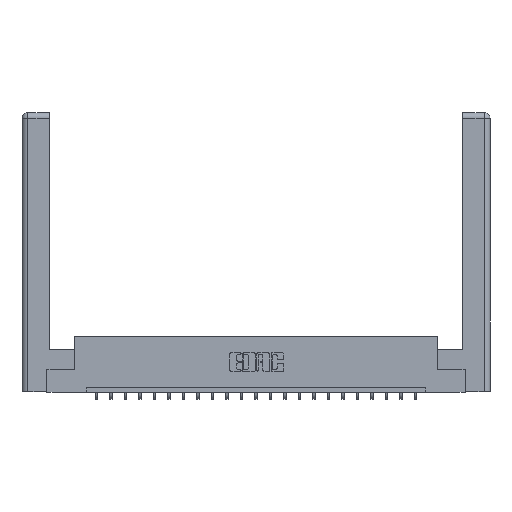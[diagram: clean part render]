
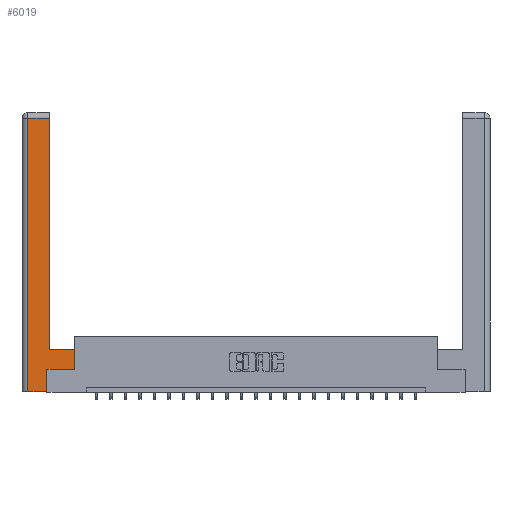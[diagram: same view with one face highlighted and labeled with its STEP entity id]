
A CAD part, top view. The second image highlights one B-rep face of the part: STEP entity #6019.
In plain terms, the highlighted planar face has unit normal (0, 0, 1).
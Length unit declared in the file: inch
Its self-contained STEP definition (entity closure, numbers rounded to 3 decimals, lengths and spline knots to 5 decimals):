
#925 = CARTESIAN_POINT ( 'NONE',  ( 0., 0., 0. ) ) ;
#1582 = EDGE_CURVE ( 'NONE', #2678, #2414, #10447, .T. ) ;
#1807 = ORIENTED_EDGE ( 'NONE', *, *, #10558, .T. ) ;
#2045 = CARTESIAN_POINT ( 'NONE',  ( 0.295, 0.45, 0. ) ) ;
#2333 = VECTOR ( 'NONE', #15554, 39.37008 ) ;
#2414 = VERTEX_POINT ( 'NONE', #6333 ) ;
#2653 = EDGE_CURVE ( 'NONE', #2414, #18316, #16568, .T. ) ;
#2678 = VERTEX_POINT ( 'NONE', #7148 ) ;
#3424 = DIRECTION ( 'NONE',  ( 0., 1., 0. ) ) ;
#3542 = CARTESIAN_POINT ( 'NONE',  ( 0.295, 0.45, 0. ) ) ;
#3583 = DIRECTION ( 'NONE',  ( -1., 0., 0. ) ) ;
#4177 = LINE ( 'NONE', #17579, #14940 ) ;
#4612 = LINE ( 'NONE', #7043, #17806 ) ;
#5294 = EDGE_CURVE ( 'NONE', #15236, #6490, #16550, .T. ) ;
#5371 = EDGE_CURVE ( 'NONE', #18316, #11272, #4177, .T. ) ;
#6019 = ADVANCED_FACE ( 'NONE', ( #17327 ), #9470, .F. ) ;
#6333 = CARTESIAN_POINT ( 'NONE',  ( 0.565, 0.45, 0. ) ) ;
#6456 = ORIENTED_EDGE ( 'NONE', *, *, #5294, .T. ) ;
#6490 = VERTEX_POINT ( 'NONE', #19082 ) ;
#7034 = ORIENTED_EDGE ( 'NONE', *, *, #5371, .T. ) ;
#7043 = CARTESIAN_POINT ( 'NONE',  ( 0.565, 0.245, 0. ) ) ;
#7148 = CARTESIAN_POINT ( 'NONE',  ( 0.565, 0.245, 0. ) ) ;
#7557 = EDGE_CURVE ( 'NONE', #6490, #10489, #11577, .T. ) ;
#7897 = DIRECTION ( 'NONE',  ( -1., 0., 0. ) ) ;
#8452 = CARTESIAN_POINT ( 'NONE',  ( 0.0615, 2.94, 0. ) ) ;
#8713 = DIRECTION ( 'NONE',  ( 1., 0., 0. ) ) ;
#8998 = LINE ( 'NONE', #10266, #11144 ) ;
#9437 = VECTOR ( 'NONE', #15833, 39.37008 ) ;
#9470 = PLANE ( 'NONE',  #16170 ) ;
#10266 = CARTESIAN_POINT ( 'NONE',  ( 0.0615, 2.94, 0. ) ) ;
#10368 = VECTOR ( 'NONE', #16097, 39.37008 ) ;
#10447 = LINE ( 'NONE', #20056, #20625 ) ;
#10489 = VERTEX_POINT ( 'NONE', #15449 ) ;
#10558 = EDGE_CURVE ( 'NONE', #11272, #13609, #8998, .T. ) ;
#11144 = VECTOR ( 'NONE', #3583, 39.37008 ) ;
#11272 = VERTEX_POINT ( 'NONE', #19747 ) ;
#11407 = ORIENTED_EDGE ( 'NONE', *, *, #16576, .T. ) ;
#11577 = LINE ( 'NONE', #21186, #9437 ) ;
#13609 = VERTEX_POINT ( 'NONE', #8452 ) ;
#14940 = VECTOR ( 'NONE', #21042, 39.37008 ) ;
#15011 = DIRECTION ( 'NONE',  ( 0., -1., 0. ) ) ;
#15236 = VERTEX_POINT ( 'NONE', #18381 ) ;
#15449 = CARTESIAN_POINT ( 'NONE',  ( 0.265, 0.245, 0. ) ) ;
#15554 = DIRECTION ( 'NONE',  ( -1., 0., 0. ) ) ;
#15833 = DIRECTION ( 'NONE',  ( 0., 1., 0. ) ) ;
#15844 = EDGE_CURVE ( 'NONE', #10489, #2678, #4612, .T. ) ;
#16097 = DIRECTION ( 'NONE',  ( 1., 0., 0. ) ) ;
#16170 = AXIS2_PLACEMENT_3D ( 'NONE', #925, #21529, #7897 ) ;
#16186 = ORIENTED_EDGE ( 'NONE', *, *, #2653, .T. ) ;
#16550 = LINE ( 'NONE', #18359, #10368 ) ;
#16568 = LINE ( 'NONE', #3542, #2333 ) ;
#16576 = EDGE_CURVE ( 'NONE', #13609, #15236, #21809, .T. ) ;
#17061 = ORIENTED_EDGE ( 'NONE', *, *, #1582, .T. ) ;
#17327 = FACE_OUTER_BOUND ( 'NONE', #22141, .T. ) ;
#17457 = ORIENTED_EDGE ( 'NONE', *, *, #7557, .T. ) ;
#17579 = CARTESIAN_POINT ( 'NONE',  ( 0.295, 3., 0. ) ) ;
#17806 = VECTOR ( 'NONE', #8713, 39.37008 ) ;
#18316 = VERTEX_POINT ( 'NONE', #2045 ) ;
#18359 = CARTESIAN_POINT ( 'NONE',  ( 0.265, 0., 0. ) ) ;
#18381 = CARTESIAN_POINT ( 'NONE',  ( 0.0615, 0., 0. ) ) ;
#18544 = CARTESIAN_POINT ( 'NONE',  ( 0.0615, 0., 0. ) ) ;
#19082 = CARTESIAN_POINT ( 'NONE',  ( 0.265, 0., 0. ) ) ;
#19747 = CARTESIAN_POINT ( 'NONE',  ( 0.295, 2.94, 0. ) ) ;
#20056 = CARTESIAN_POINT ( 'NONE',  ( 0.565, 0.45, 0. ) ) ;
#20625 = VECTOR ( 'NONE', #3424, 39.37008 ) ;
#21042 = DIRECTION ( 'NONE',  ( 0., 1., 0. ) ) ;
#21186 = CARTESIAN_POINT ( 'NONE',  ( 0.265, 0.245, 0. ) ) ;
#21259 = VECTOR ( 'NONE', #15011, 39.37008 ) ;
#21529 = DIRECTION ( 'NONE',  ( 0., 0., -1. ) ) ;
#21809 = LINE ( 'NONE', #18544, #21259 ) ;
#22141 = EDGE_LOOP ( 'NONE', ( #7034, #1807, #11407, #6456, #17457, #22219, #17061, #16186 ) ) ;
#22219 = ORIENTED_EDGE ( 'NONE', *, *, #15844, .T. ) ;
